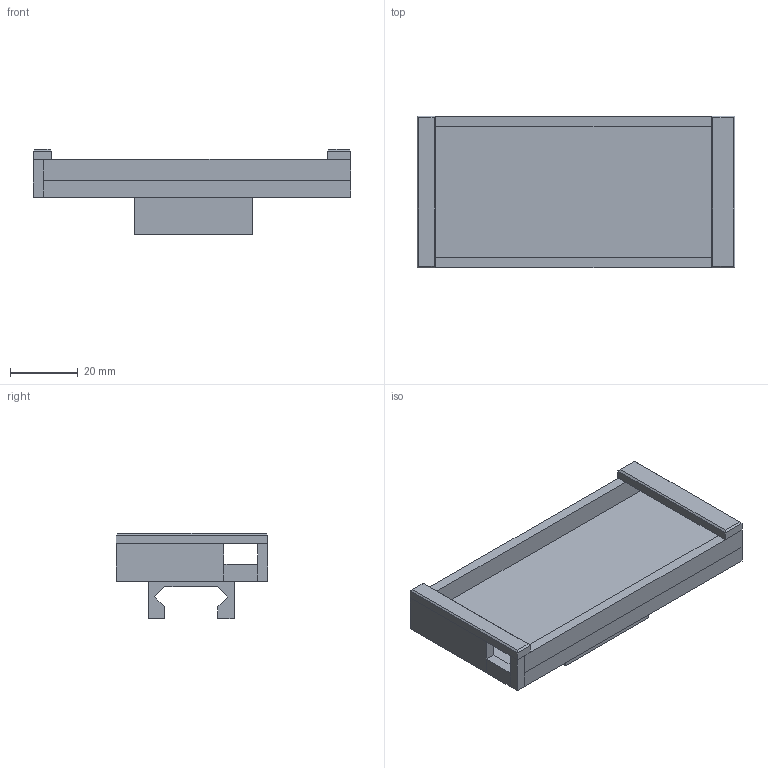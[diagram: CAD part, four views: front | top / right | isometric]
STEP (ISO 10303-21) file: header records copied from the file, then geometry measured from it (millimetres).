
FILE_DESCRIPTION(('Open CASCADE Model'),'2;1');
FILE_NAME('Open CASCADE Shape Model','2013-08-15T17:39:55',('Author'),( 'Open CASCADE'),'Open CASCADE STEP processor 6.5','Open CASCADE 6.5' ,'Unknown');
FILE_SCHEMA(('AUTOMOTIVE_DESIGN_CC2 { 1 2 10303 214 -1 1 5 4 }'));
Length unit declared in the file: millimetre
Products named in the file (1): IpodNano4gPicatinny
Bounding box: 94 x 44.9 x 25.24 mm (x, y, z)
Volume: 30773.4 mm3; surface area: 15764.9 mm2
Topology: 1 solids, 1 shells, 63 faces, 155 edges, 91 vertices
Faces by surface type: plane 63
Entity records: 3817 total; most frequent: CARTESIAN_POINT 620, DIRECTION 593, LINE 465, VECTOR 465, ORIENTED_EDGE 310, PCURVE 310, DEFINITIONAL_REPRESENTATION 310, EDGE_CURVE 155
